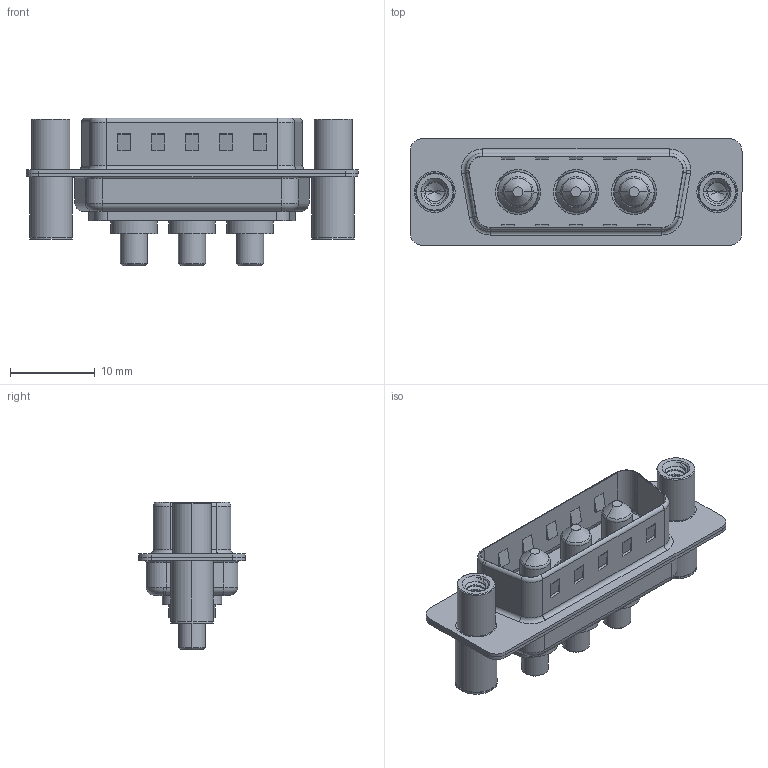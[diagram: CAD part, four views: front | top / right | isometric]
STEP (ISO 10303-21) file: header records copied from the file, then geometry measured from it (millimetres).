
FILE_DESCRIPTION (( 'STEP AP203' ), '1' );
FILE_NAME ('627-3W3-224-3T4.STEP', '2019-05-24T14:32:29', ( '' ), ( '' ), 'SwSTEP 2.0', 'SolidWorks 2016', '' );
FILE_SCHEMA (( 'CONFIG_CONTROL_DESIGN' ));
Length unit declared in the file: millimetre
Products named in the file (6): 627-3W3-224-3T4; 627Combo Housing_3W3; 627Combo Shell Rear_15 Contacts; 627Combo Shell Front_15 Contacts; 627Combo Threaded Standoff and Board Spacer_4; Power Pin_30A S
Assembly tree (8 placements, depth 2):
  627-3W3-224-3T4
    627Combo Housing_3W3
    627Combo Shell Rear_15 Contacts
    627Combo Shell Front_15 Contacts
    627Combo Threaded Standoff and Board Spacer_4  x2
    Power Pin_30A S  x3
Bounding box: 39.15 x 12.6 x 17.4 mm (x, y, z)
Volume: 2357.5 mm3; surface area: 5249.6 mm2
Topology: 11 solids, 11 shells, 546 faces, 1338 edges, 832 vertices
Faces by surface type: cylinder 242, plane 175, torus 60, cone 51, bspline 18
Entity records: 14677 total; most frequent: CARTESIAN_POINT 4387, DIRECTION 2059, ORIENTED_EDGE 1984, EDGE_CURVE 992, AXIS2_PLACEMENT_3D 768, VERTEX_POINT 623, LINE 523, VECTOR 523
